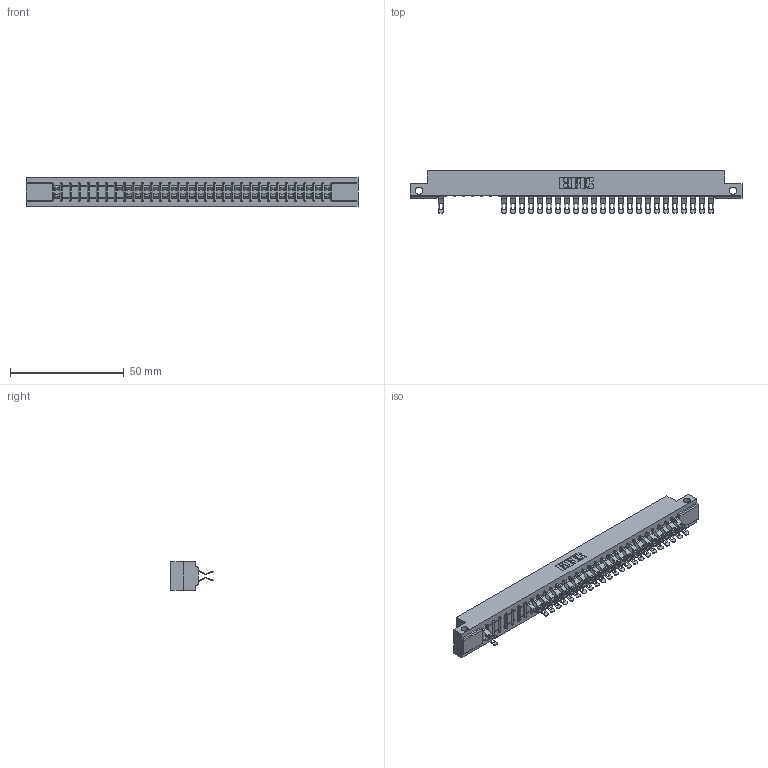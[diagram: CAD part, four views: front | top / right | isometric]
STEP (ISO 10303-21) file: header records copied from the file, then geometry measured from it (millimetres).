
FILE_DESCRIPTION (( 'STEP AP203' ), '1' );
FILE_NAME ('307-062-555-212.STEP', '2018-08-06T09:28:17', ( '' ), ( '' ), 'SwSTEP 2.0', 'SolidWorks 2016', '' );
FILE_SCHEMA (( 'CONFIG_CONTROL_DESIGN' ));
Length unit declared in the file: inch
Products named in the file (3): 307 Part_.128 Dia Side Mounting Holes; 307-290-001_555; 307-062-555-212
Assembly tree (50 placements, depth 2):
  307-062-555-212
    307 Part_.128 Dia Side Mounting Holes
    307-290-001_555  x49
Bounding box: 145.85 x 18.75 x 12.7 mm (x, y, z)
Volume: 15266.7 mm3; surface area: 18148.2 mm2
Topology: 50 solids, 50 shells, 3269 faces, 9608 edges, 6252 vertices
Faces by surface type: plane 1814, cylinder 1391, sphere 64
Entity records: 29047 total; most frequent: CARTESIAN_POINT 4814, ORIENTED_EDGE 4784, DIRECTION 4714, EDGE_CURVE 2392, VECTOR 1818, LINE 1818, VERTEX_POINT 1548, AXIS2_PLACEMENT_3D 1448
